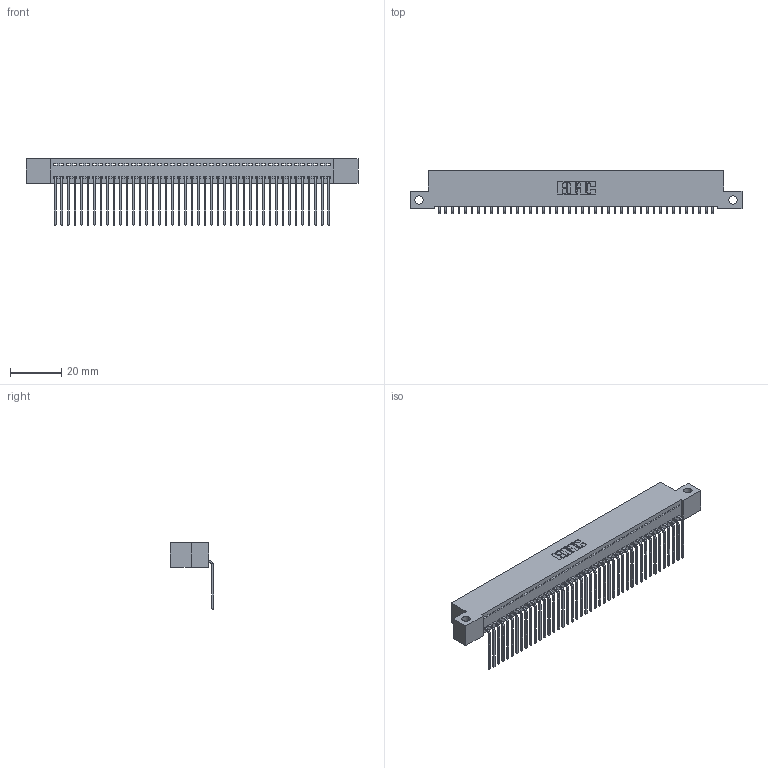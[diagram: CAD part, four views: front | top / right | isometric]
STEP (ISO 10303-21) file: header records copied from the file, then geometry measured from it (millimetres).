
FILE_DESCRIPTION (( 'STEP AP203' ), '1' );
FILE_NAME ('342-043-559-112.STEP', '2019-10-02T18:47:04', ( '' ), ( '' ), 'SwSTEP 2.0', 'SolidWorks 2016', '' );
FILE_SCHEMA (( 'CONFIG_CONTROL_DESIGN' ));
Length unit declared in the file: inch
Products named in the file (3): 342 Part_Side Mount; 345-292-001_558 559 Tail - 1; 342-043-559-112
Assembly tree (44 placements, depth 2):
  342-043-559-112
    342 Part_Side Mount
    345-292-001_558 559 Tail - 1  x43
Bounding box: 129.54 x 16.83 x 25.78 mm (x, y, z)
Volume: 11431.1 mm3; surface area: 17455.3 mm2
Topology: 44 solids, 44 shells, 2690 faces, 8125 edges, 5358 vertices
Faces by surface type: plane 1958, cylinder 732
Entity records: 26113 total; most frequent: CARTESIAN_POINT 4511, ORIENTED_EDGE 4490, DIRECTION 3803, EDGE_CURVE 2245, LINE 2117, VECTOR 2117, VERTEX_POINT 1494, AXIS2_PLACEMENT_3D 843
